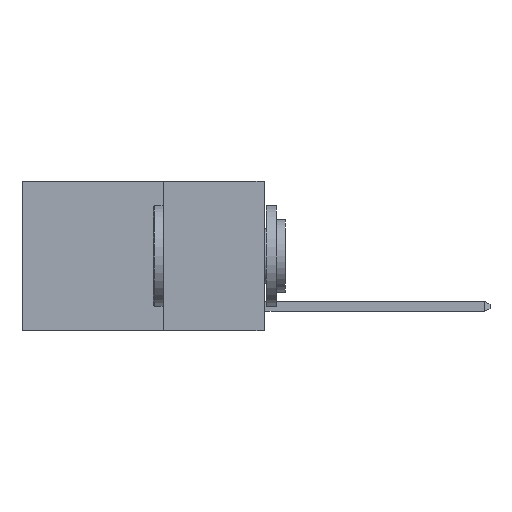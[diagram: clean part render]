
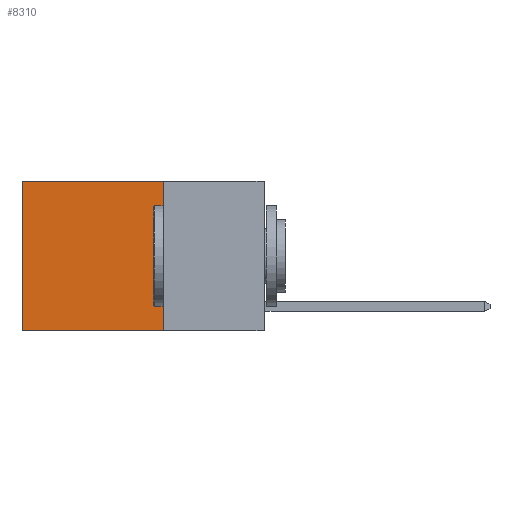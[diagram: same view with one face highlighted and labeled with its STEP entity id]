
A CAD part, left-side view. The second image highlights one B-rep face of the part: STEP entity #8310.
In plain terms, the highlighted planar face has unit normal (-1, 0, 0).
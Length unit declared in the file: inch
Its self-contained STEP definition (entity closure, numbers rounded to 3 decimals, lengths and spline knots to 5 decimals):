
#253 = ORIENTED_EDGE ( 'NONE', *, *, #3195, .F. ) ;
#566 = VECTOR ( 'NONE', #2885, 39.37008 ) ;
#1693 = ORIENTED_EDGE ( 'NONE', *, *, #3832, .F. ) ;
#1754 = DIRECTION ( 'NONE',  ( 0., 0., -1. ) ) ;
#2124 = CARTESIAN_POINT ( 'NONE',  ( 0.2625, 0.25, -0.37 ) ) ;
#2326 = ORIENTED_EDGE ( 'NONE', *, *, #5370, .T. ) ;
#2730 = CARTESIAN_POINT ( 'NONE',  ( 0.2625, 0.25, 0. ) ) ;
#2885 = DIRECTION ( 'NONE',  ( 0., 0., -1. ) ) ;
#3195 = EDGE_CURVE ( 'NONE', #5872, #4763, #8682, .T. ) ;
#3284 = VECTOR ( 'NONE', #6164, 39.37008 ) ;
#3832 = EDGE_CURVE ( 'NONE', #4763, #10249, #3839, .T. ) ;
#3839 = LINE ( 'NONE', #2124, #10967 ) ;
#4230 = VERTEX_POINT ( 'NONE', #12052 ) ;
#4364 = AXIS2_PLACEMENT_3D ( 'NONE', #12026, #7401, #1754 ) ;
#4763 = VERTEX_POINT ( 'NONE', #5282 ) ;
#4955 = FACE_OUTER_BOUND ( 'NONE', #10896, .T. ) ;
#5282 = CARTESIAN_POINT ( 'NONE',  ( 0.2625, 0.25, -0.37 ) ) ;
#5370 = EDGE_CURVE ( 'NONE', #5872, #4230, #6058, .T. ) ;
#5872 = VERTEX_POINT ( 'NONE', #2730 ) ;
#6058 = LINE ( 'NONE', #9845, #3284 ) ;
#6092 = CARTESIAN_POINT ( 'NONE',  ( 0.2625, 0.6, -0.37 ) ) ;
#6164 = DIRECTION ( 'NONE',  ( 0., 1., 0. ) ) ;
#6462 = PLANE ( 'NONE',  #4364 ) ;
#7401 = DIRECTION ( 'NONE',  ( 1., 0., 0. ) ) ;
#7524 = DIRECTION ( 'NONE',  ( 0., 0., -1. ) ) ;
#7607 = VECTOR ( 'NONE', #7524, 39.37008 ) ;
#8310 = ADVANCED_FACE ( 'NONE', ( #4955 ), #6462, .F. ) ;
#8682 = LINE ( 'NONE', #11298, #566 ) ;
#9183 = ORIENTED_EDGE ( 'NONE', *, *, #12104, .T. ) ;
#9845 = CARTESIAN_POINT ( 'NONE',  ( 0.2625, 0.25, 0. ) ) ;
#10249 = VERTEX_POINT ( 'NONE', #6092 ) ;
#10357 = LINE ( 'NONE', #11209, #7607 ) ;
#10896 = EDGE_LOOP ( 'NONE', ( #9183, #1693, #253, #2326 ) ) ;
#10967 = VECTOR ( 'NONE', #11481, 39.37008 ) ;
#11209 = CARTESIAN_POINT ( 'NONE',  ( 0.2625, 0.6, 0. ) ) ;
#11298 = CARTESIAN_POINT ( 'NONE',  ( 0.2625, 0.25, 0. ) ) ;
#11481 = DIRECTION ( 'NONE',  ( 0., 1., 0. ) ) ;
#12026 = CARTESIAN_POINT ( 'NONE',  ( 0.2625, 0.25, 0. ) ) ;
#12052 = CARTESIAN_POINT ( 'NONE',  ( 0.2625, 0.6, 0. ) ) ;
#12104 = EDGE_CURVE ( 'NONE', #4230, #10249, #10357, .T. ) ;
